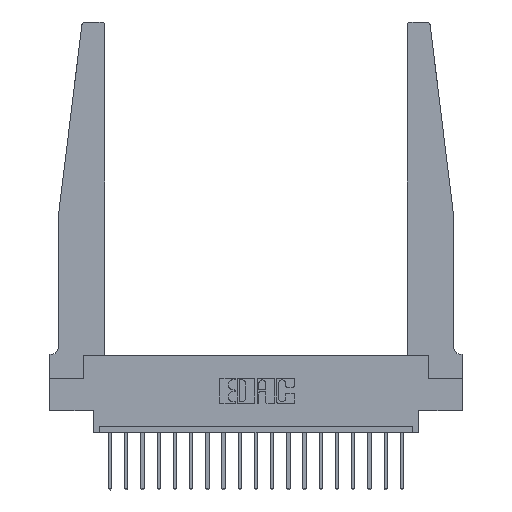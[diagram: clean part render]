
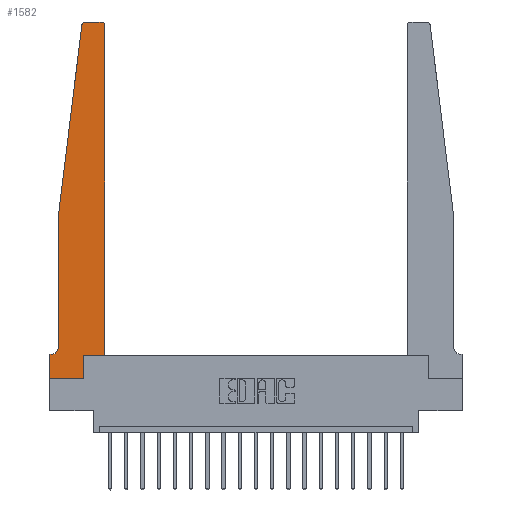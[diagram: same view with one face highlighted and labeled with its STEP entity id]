
A CAD part, top view. The second image highlights one B-rep face of the part: STEP entity #1582.
In plain terms, the highlighted planar face has unit normal (0, 0, 1).
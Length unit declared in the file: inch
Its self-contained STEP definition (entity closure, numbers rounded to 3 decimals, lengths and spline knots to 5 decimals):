
#36 = VECTOR ( 'NONE', #1225, 39.37008 ) ;
#444 = ORIENTED_EDGE ( 'NONE', *, *, #15024, .T. ) ;
#638 = DIRECTION ( 'NONE',  ( 1., 0., 0. ) ) ;
#711 = AXIS2_PLACEMENT_3D ( 'NONE', #8824, #4283, #14961 ) ;
#964 = VERTEX_POINT ( 'NONE', #18363 ) ;
#1225 = DIRECTION ( 'NONE',  ( 1., 0., 0. ) ) ;
#1268 = EDGE_CURVE ( 'NONE', #8039, #17058, #8112, .T. ) ;
#1535 = LINE ( 'NONE', #3678, #19448 ) ;
#1549 = PLANE ( 'NONE',  #7057 ) ;
#1582 = ADVANCED_FACE ( 'NONE', ( #16254 ), #1549, .T. ) ;
#1613 = VECTOR ( 'NONE', #8655, 39.37008 ) ;
#1719 = CARTESIAN_POINT ( 'NONE',  ( 0.015, 0.1875, 0.37 ) ) ;
#1772 = ORIENTED_EDGE ( 'NONE', *, *, #2683, .T. ) ;
#1797 = CARTESIAN_POINT ( 'NONE',  ( 0.425, 0.18, 0.37 ) ) ;
#1954 = EDGE_LOOP ( 'NONE', ( #14959, #3651, #6817, #17413, #1772, #15527, #3354, #16229, #8476, #12675, #15918, #444 ) ) ;
#2055 = AXIS2_PLACEMENT_3D ( 'NONE', #17985, #19584, #10381 ) ;
#2683 = EDGE_CURVE ( 'NONE', #15610, #7113, #16920, .T. ) ;
#2691 = CARTESIAN_POINT ( 'NONE',  ( 0.065, 0.1875, 0.37 ) ) ;
#3143 = EDGE_CURVE ( 'NONE', #5010, #15610, #16155, .T. ) ;
#3354 = ORIENTED_EDGE ( 'NONE', *, *, #18842, .T. ) ;
#3651 = ORIENTED_EDGE ( 'NONE', *, *, #8292, .T. ) ;
#3678 = CARTESIAN_POINT ( 'NONE',  ( 0.425, 0.18, 0.37 ) ) ;
#3733 = EDGE_CURVE ( 'NONE', #7113, #8169, #16904, .T. ) ;
#3753 = DIRECTION ( 'NONE',  ( -0.122, -0.992, 0. ) ) ;
#4105 = AXIS2_PLACEMENT_3D ( 'NONE', #4738, #15443, #16998 ) ;
#4198 = CARTESIAN_POINT ( 'NONE',  ( 0.425, 0.18, 0.37 ) ) ;
#4283 = DIRECTION ( 'NONE',  ( 0., 0., -1. ) ) ;
#4377 = VERTEX_POINT ( 'NONE', #6696 ) ;
#4738 = CARTESIAN_POINT ( 'NONE',  ( 0.27653, 2.72, 0.37 ) ) ;
#4981 = DIRECTION ( 'NONE',  ( 0., -1., 0. ) ) ;
#5010 = VERTEX_POINT ( 'NONE', #9945 ) ;
#6197 = EDGE_CURVE ( 'NONE', #10825, #8039, #14886, .T. ) ;
#6406 = LINE ( 'NONE', #18067, #15247 ) ;
#6696 = CARTESIAN_POINT ( 'NONE',  ( 0.24675, 2.72367, 0.37 ) ) ;
#6742 = CARTESIAN_POINT ( 'NONE',  ( 0.065, 1.25, 0.37 ) ) ;
#6817 = ORIENTED_EDGE ( 'NONE', *, *, #9879, .T. ) ;
#7057 = AXIS2_PLACEMENT_3D ( 'NONE', #15720, #12712, #17289 ) ;
#7113 = VERTEX_POINT ( 'NONE', #1719 ) ;
#7749 = LINE ( 'NONE', #8093, #13757 ) ;
#8004 = CARTESIAN_POINT ( 'NONE',  ( 0.2605, 0.18, 0.37 ) ) ;
#8039 = VERTEX_POINT ( 'NONE', #8004 ) ;
#8065 = EDGE_CURVE ( 'NONE', #8752, #10825, #19357, .T. ) ;
#8087 = CIRCLE ( 'NONE', #2055, 0.03 ) ;
#8093 = CARTESIAN_POINT ( 'NONE',  ( 0., 0., 0.37 ) ) ;
#8112 = LINE ( 'NONE', #4198, #36 ) ;
#8169 = VERTEX_POINT ( 'NONE', #12722 ) ;
#8292 = EDGE_CURVE ( 'NONE', #12748, #4377, #9523, .T. ) ;
#8476 = ORIENTED_EDGE ( 'NONE', *, *, #6197, .T. ) ;
#8655 = DIRECTION ( 'NONE',  ( 0., -1., 0. ) ) ;
#8752 = VERTEX_POINT ( 'NONE', #13166 ) ;
#8824 = CARTESIAN_POINT ( 'NONE',  ( 0.015, 0.2375, 0.37 ) ) ;
#8950 = CARTESIAN_POINT ( 'NONE',  ( 0.2605, 0.18, 0.37 ) ) ;
#9382 = VECTOR ( 'NONE', #16454, 39.37008 ) ;
#9398 = EDGE_CURVE ( 'NONE', #964, #12748, #6406, .T. ) ;
#9523 = CIRCLE ( 'NONE', #4105, 0.03 ) ;
#9879 = EDGE_CURVE ( 'NONE', #4377, #5010, #13316, .T. ) ;
#9945 = CARTESIAN_POINT ( 'NONE',  ( 0.065, 1.25, 0.37 ) ) ;
#10381 = DIRECTION ( 'NONE',  ( 1., 0., 0. ) ) ;
#10825 = VERTEX_POINT ( 'NONE', #16633 ) ;
#11343 = VECTOR ( 'NONE', #19778, 39.37008 ) ;
#11577 = CARTESIAN_POINT ( 'NONE',  ( 0.065, 1.25, 0.37 ) ) ;
#12244 = CARTESIAN_POINT ( 'NONE',  ( 0., 0., 0.37 ) ) ;
#12675 = ORIENTED_EDGE ( 'NONE', *, *, #1268, .T. ) ;
#12712 = DIRECTION ( 'NONE',  ( 0., 0., 1. ) ) ;
#12722 = CARTESIAN_POINT ( 'NONE',  ( 0., 0.1875, 0.37 ) ) ;
#12748 = VERTEX_POINT ( 'NONE', #15230 ) ;
#13166 = CARTESIAN_POINT ( 'NONE',  ( 0., 0., 0.37 ) ) ;
#13316 = LINE ( 'NONE', #6742, #13552 ) ;
#13473 = EDGE_CURVE ( 'NONE', #17058, #18600, #1535, .T. ) ;
#13552 = VECTOR ( 'NONE', #3753, 39.37008 ) ;
#13757 = VECTOR ( 'NONE', #4981, 39.37008 ) ;
#14886 = LINE ( 'NONE', #8950, #9382 ) ;
#14959 = ORIENTED_EDGE ( 'NONE', *, *, #9398, .T. ) ;
#14961 = DIRECTION ( 'NONE',  ( -1., 0., 0. ) ) ;
#14994 = CARTESIAN_POINT ( 'NONE',  ( 0.065, 0.2375, 0.37 ) ) ;
#15024 = EDGE_CURVE ( 'NONE', #18600, #964, #8087, .T. ) ;
#15230 = CARTESIAN_POINT ( 'NONE',  ( 0.27653, 2.75, 0.37 ) ) ;
#15247 = VECTOR ( 'NONE', #19741, 39.37008 ) ;
#15443 = DIRECTION ( 'NONE',  ( 0., 0., 1. ) ) ;
#15527 = ORIENTED_EDGE ( 'NONE', *, *, #3733, .T. ) ;
#15610 = VERTEX_POINT ( 'NONE', #14994 ) ;
#15720 = CARTESIAN_POINT ( 'NONE',  ( 0., 0.1875, 0.37 ) ) ;
#15918 = ORIENTED_EDGE ( 'NONE', *, *, #13473, .T. ) ;
#16155 = LINE ( 'NONE', #11577, #1613 ) ;
#16229 = ORIENTED_EDGE ( 'NONE', *, *, #8065, .T. ) ;
#16254 = FACE_OUTER_BOUND ( 'NONE', #1954, .T. ) ;
#16454 = DIRECTION ( 'NONE',  ( 0., 1., 0. ) ) ;
#16633 = CARTESIAN_POINT ( 'NONE',  ( 0.2605, 0., 0.37 ) ) ;
#16772 = CARTESIAN_POINT ( 'NONE',  ( 0.425, 2.72, 0.37 ) ) ;
#16904 = LINE ( 'NONE', #2691, #11343 ) ;
#16920 = CIRCLE ( 'NONE', #711, 0.05 ) ;
#16998 = DIRECTION ( 'NONE',  ( 1., 0., 0. ) ) ;
#17058 = VERTEX_POINT ( 'NONE', #1797 ) ;
#17289 = DIRECTION ( 'NONE',  ( 1., 0., 0. ) ) ;
#17413 = ORIENTED_EDGE ( 'NONE', *, *, #3143, .T. ) ;
#17560 = DIRECTION ( 'NONE',  ( 0., 1., 0. ) ) ;
#17985 = CARTESIAN_POINT ( 'NONE',  ( 0.395, 2.72, 0.37 ) ) ;
#18067 = CARTESIAN_POINT ( 'NONE',  ( 0.25, 2.75, 0.37 ) ) ;
#18179 = VECTOR ( 'NONE', #638, 39.37008 ) ;
#18363 = CARTESIAN_POINT ( 'NONE',  ( 0.395, 2.75, 0.37 ) ) ;
#18600 = VERTEX_POINT ( 'NONE', #16772 ) ;
#18842 = EDGE_CURVE ( 'NONE', #8169, #8752, #7749, .T. ) ;
#19357 = LINE ( 'NONE', #12244, #18179 ) ;
#19448 = VECTOR ( 'NONE', #17560, 39.37008 ) ;
#19584 = DIRECTION ( 'NONE',  ( 0., 0., 1. ) ) ;
#19741 = DIRECTION ( 'NONE',  ( -1., 0., 0. ) ) ;
#19778 = DIRECTION ( 'NONE',  ( -1., 0., 0. ) ) ;
